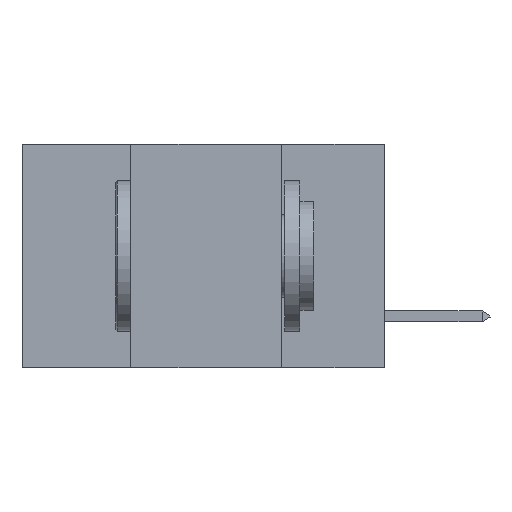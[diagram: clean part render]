
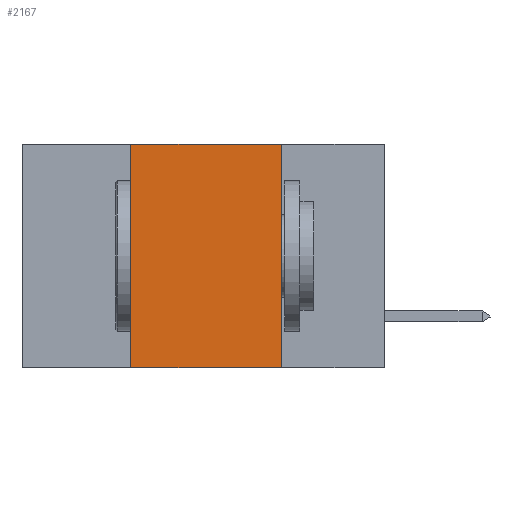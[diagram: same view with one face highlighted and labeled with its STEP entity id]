
A CAD part, left-side view. The second image highlights one B-rep face of the part: STEP entity #2167.
In plain terms, the highlighted planar face has unit normal (-1, 0, 0).
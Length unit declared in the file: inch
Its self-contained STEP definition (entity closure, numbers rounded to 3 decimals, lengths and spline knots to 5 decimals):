
#34 = VECTOR ( 'NONE', #25576, 39.37008 ) ;
#1266 = CARTESIAN_POINT ( 'NONE',  ( 0., 0.6, -0.37 ) ) ;
#1512 = ORIENTED_EDGE ( 'NONE', *, *, #2357, .F. ) ;
#2167 = ADVANCED_FACE ( 'NONE', ( #9721 ), #4041, .F. ) ;
#2357 = EDGE_CURVE ( 'NONE', #19758, #9193, #16578, .T. ) ;
#2461 = DIRECTION ( 'NONE',  ( 0., 0., -1. ) ) ;
#2604 = AXIS2_PLACEMENT_3D ( 'NONE', #22203, #8417, #19099 ) ;
#3969 = ORIENTED_EDGE ( 'NONE', *, *, #27376, .F. ) ;
#4041 = PLANE ( 'NONE',  #2604 ) ;
#5000 = CARTESIAN_POINT ( 'NONE',  ( 0., 0.17, 0. ) ) ;
#8417 = DIRECTION ( 'NONE',  ( 1., 0., 0. ) ) ;
#8771 = CARTESIAN_POINT ( 'NONE',  ( 0., 0.17, 0. ) ) ;
#9193 = VERTEX_POINT ( 'NONE', #22903 ) ;
#9721 = FACE_OUTER_BOUND ( 'NONE', #27188, .T. ) ;
#12530 = CARTESIAN_POINT ( 'NONE',  ( 0., 0.6, 0. ) ) ;
#13174 = LINE ( 'NONE', #18711, #15127 ) ;
#14317 = VECTOR ( 'NONE', #2461, 39.37008 ) ;
#14396 = VERTEX_POINT ( 'NONE', #28124 ) ;
#15127 = VECTOR ( 'NONE', #29563, 39.37008 ) ;
#16578 = LINE ( 'NONE', #5000, #14317 ) ;
#17826 = EDGE_CURVE ( 'NONE', #14396, #9193, #25751, .T. ) ;
#18563 = CARTESIAN_POINT ( 'NONE',  ( 0., 0.42, 0. ) ) ;
#18711 = CARTESIAN_POINT ( 'NONE',  ( 0., 0.42, 0. ) ) ;
#19099 = DIRECTION ( 'NONE',  ( 0., 0., -1. ) ) ;
#19758 = VERTEX_POINT ( 'NONE', #8771 ) ;
#19808 = ORIENTED_EDGE ( 'NONE', *, *, #17826, .T. ) ;
#22203 = CARTESIAN_POINT ( 'NONE',  ( 0., 0.6, 0. ) ) ;
#22323 = DIRECTION ( 'NONE',  ( 0., -1., 0. ) ) ;
#22903 = CARTESIAN_POINT ( 'NONE',  ( 0., 0.17, -0.37 ) ) ;
#23481 = LINE ( 'NONE', #12530, #30654 ) ;
#25576 = DIRECTION ( 'NONE',  ( 0., -1., 0. ) ) ;
#25751 = LINE ( 'NONE', #1266, #34 ) ;
#27188 = EDGE_LOOP ( 'NONE', ( #1512, #30456, #3969, #19808 ) ) ;
#27376 = EDGE_CURVE ( 'NONE', #14396, #30530, #13174, .T. ) ;
#27823 = EDGE_CURVE ( 'NONE', #30530, #19758, #23481, .T. ) ;
#28124 = CARTESIAN_POINT ( 'NONE',  ( 0., 0.42, -0.37 ) ) ;
#29563 = DIRECTION ( 'NONE',  ( 0., 0., 1. ) ) ;
#30456 = ORIENTED_EDGE ( 'NONE', *, *, #27823, .F. ) ;
#30530 = VERTEX_POINT ( 'NONE', #18563 ) ;
#30654 = VECTOR ( 'NONE', #22323, 39.37008 ) ;
